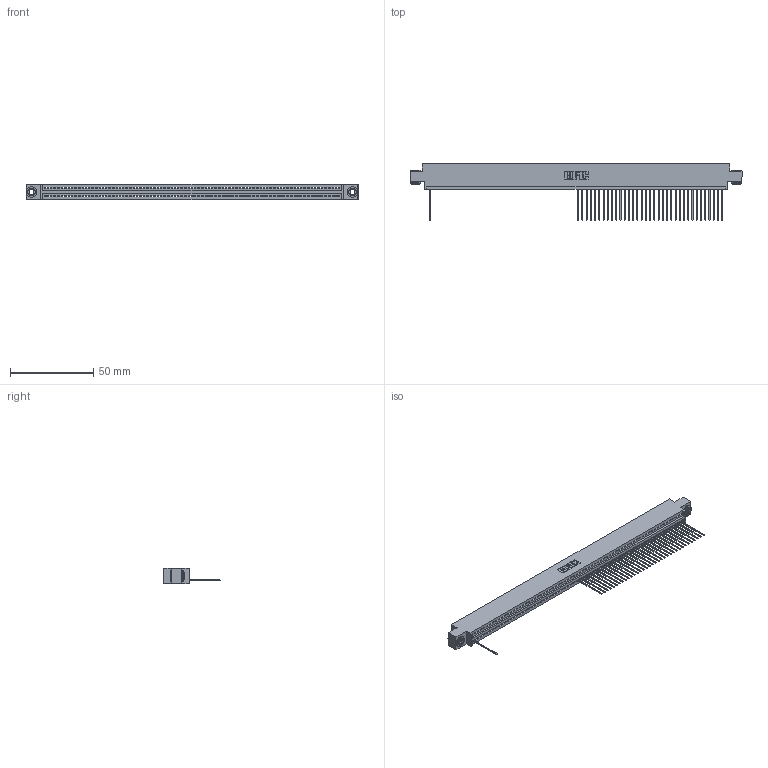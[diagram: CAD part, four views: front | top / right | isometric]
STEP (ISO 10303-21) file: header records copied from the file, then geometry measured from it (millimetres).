
FILE_DESCRIPTION (( 'STEP AP203' ), '1' );
FILE_NAME ('395-070-541-603.STEP', '2018-11-26T20:05:34', ( '' ), ( '' ), 'SwSTEP 2.0', 'SolidWorks 2016', '' );
FILE_SCHEMA (( 'CONFIG_CONTROL_DESIGN' ));
Length unit declared in the file: inch
Products named in the file (4): 345-250-002_345-250-002-102; 345-292-001_345-293-141; 345 Part_0.170 Offset - 0.156 Dia-TH; 395-070-541-603
Assembly tree (39 placements, depth 2):
  395-070-541-603
    345 Part_0.170 Offset - 0.156 Dia-TH
    345-292-001_345-293-141  x36
    345-250-002_345-250-002-102  x2
Bounding box: 199.01 x 33.96 x 9.4 mm (x, y, z)
Volume: 18766.9 mm3; surface area: 24292.6 mm2
Topology: 39 solids, 39 shells, 2800 faces, 8601 edges, 5682 vertices
Faces by surface type: plane 2010, cylinder 782, cone 8
Entity records: 48626 total; most frequent: ORIENTED_EDGE 8586, CARTESIAN_POINT 8555, DIRECTION 7423, EDGE_CURVE 4293, VECTOR 3857, LINE 3857, VERTEX_POINT 2858, AXIS2_PLACEMENT_3D 1783
